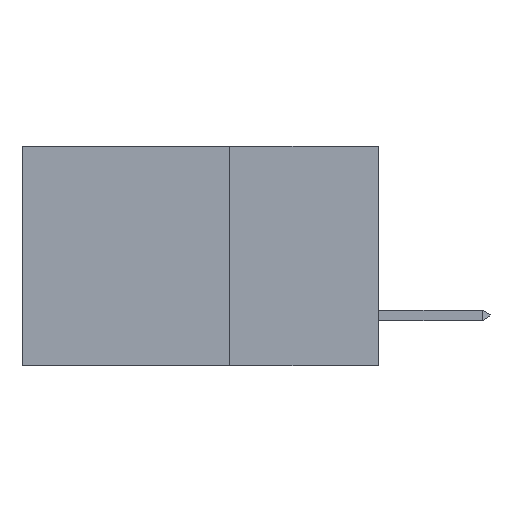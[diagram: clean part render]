
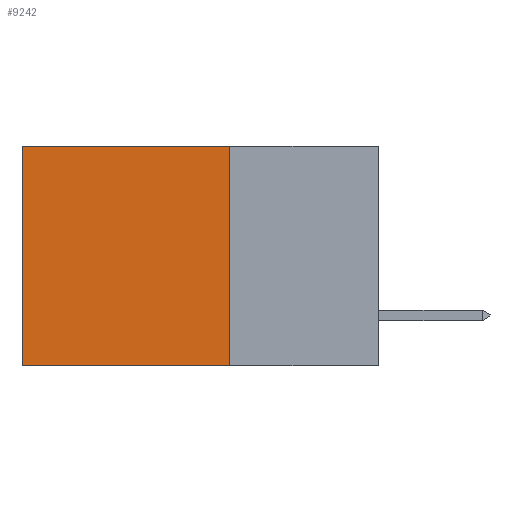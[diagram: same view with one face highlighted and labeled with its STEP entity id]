
A CAD part, left-side view. The second image highlights one B-rep face of the part: STEP entity #9242.
In plain terms, the highlighted planar face has unit normal (-1, 0, 0).
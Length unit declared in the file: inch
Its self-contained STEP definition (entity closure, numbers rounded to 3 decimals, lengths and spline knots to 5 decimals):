
#1167 = CARTESIAN_POINT ( 'NONE',  ( 0.298, 0.6, 0. ) ) ;
#1293 = DIRECTION ( 'NONE',  ( 1., 0., 0. ) ) ;
#1814 = EDGE_CURVE ( 'NONE', #14833, #10699, #1862, .T. ) ;
#1862 = LINE ( 'NONE', #10521, #6307 ) ;
#2080 = EDGE_CURVE ( 'NONE', #14833, #14813, #4810, .T. ) ;
#3946 = EDGE_CURVE ( 'NONE', #14813, #18816, #11428, .T. ) ;
#4166 = EDGE_CURVE ( 'NONE', #10699, #18816, #11126, .T. ) ;
#4810 = LINE ( 'NONE', #19888, #23832 ) ;
#5999 = FACE_OUTER_BOUND ( 'NONE', #11174, .T. ) ;
#6307 = VECTOR ( 'NONE', #18635, 39.37008 ) ;
#6784 = DIRECTION ( 'NONE',  ( 0., 0., -1. ) ) ;
#8729 = CARTESIAN_POINT ( 'NONE',  ( 0.298, 0.25, 0. ) ) ;
#9242 = ADVANCED_FACE ( 'NONE', ( #5999 ), #12464, .F. ) ;
#10521 = CARTESIAN_POINT ( 'NONE',  ( 0.298, 0.25, 0. ) ) ;
#10699 = VERTEX_POINT ( 'NONE', #19900 ) ;
#11126 = LINE ( 'NONE', #1167, #20353 ) ;
#11174 = EDGE_LOOP ( 'NONE', ( #14277, #22624, #14377, #22131 ) ) ;
#11428 = LINE ( 'NONE', #15048, #20641 ) ;
#12151 = CARTESIAN_POINT ( 'NONE',  ( 0.298, 0.6, -0.37 ) ) ;
#12423 = AXIS2_PLACEMENT_3D ( 'NONE', #8729, #1293, #14306 ) ;
#12464 = PLANE ( 'NONE',  #12423 ) ;
#12666 = CARTESIAN_POINT ( 'NONE',  ( 0.298, 0.25, 0. ) ) ;
#14277 = ORIENTED_EDGE ( 'NONE', *, *, #4166, .T. ) ;
#14306 = DIRECTION ( 'NONE',  ( 0., 0., -1. ) ) ;
#14377 = ORIENTED_EDGE ( 'NONE', *, *, #2080, .F. ) ;
#14813 = VERTEX_POINT ( 'NONE', #18104 ) ;
#14833 = VERTEX_POINT ( 'NONE', #12666 ) ;
#15048 = CARTESIAN_POINT ( 'NONE',  ( 0.298, 0.25, -0.37 ) ) ;
#16781 = DIRECTION ( 'NONE',  ( 0., 0., -1. ) ) ;
#16830 = DIRECTION ( 'NONE',  ( 0., 1., 0. ) ) ;
#18104 = CARTESIAN_POINT ( 'NONE',  ( 0.298, 0.25, -0.37 ) ) ;
#18635 = DIRECTION ( 'NONE',  ( 0., 1., 0. ) ) ;
#18816 = VERTEX_POINT ( 'NONE', #12151 ) ;
#19888 = CARTESIAN_POINT ( 'NONE',  ( 0.298, 0.25, 0. ) ) ;
#19900 = CARTESIAN_POINT ( 'NONE',  ( 0.298, 0.6, 0. ) ) ;
#20353 = VECTOR ( 'NONE', #16781, 39.37008 ) ;
#20641 = VECTOR ( 'NONE', #16830, 39.37008 ) ;
#22131 = ORIENTED_EDGE ( 'NONE', *, *, #1814, .T. ) ;
#22624 = ORIENTED_EDGE ( 'NONE', *, *, #3946, .F. ) ;
#23832 = VECTOR ( 'NONE', #6784, 39.37008 ) ;
